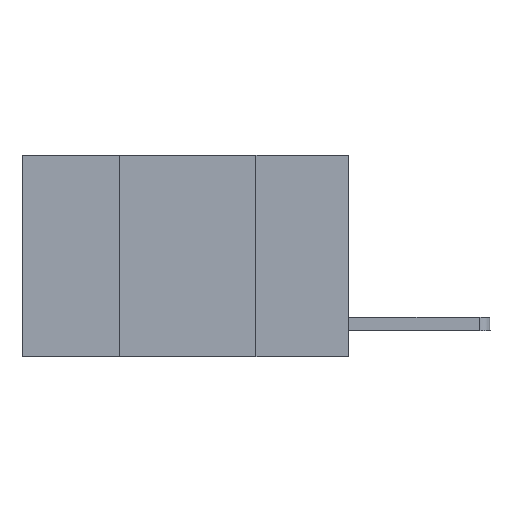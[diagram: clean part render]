
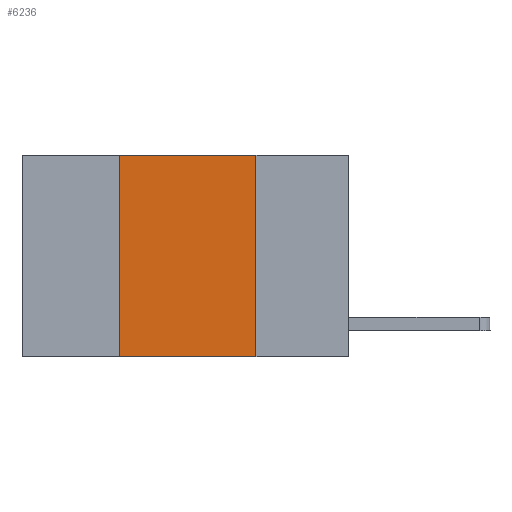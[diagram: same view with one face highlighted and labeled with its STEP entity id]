
A CAD part, left-side view. The second image highlights one B-rep face of the part: STEP entity #6236.
In plain terms, the highlighted planar face has unit normal (-1, 0, 0).
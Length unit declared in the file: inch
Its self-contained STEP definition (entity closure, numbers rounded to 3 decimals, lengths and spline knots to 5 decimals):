
#47 = EDGE_LOOP ( 'NONE', ( #7858, #4166, #7069, #5228 ) ) ;
#303 = VERTEX_POINT ( 'NONE', #2400 ) ;
#845 = DIRECTION ( 'NONE',  ( 1., 0., 0. ) ) ;
#925 = CARTESIAN_POINT ( 'NONE',  ( 0., 0.6, -0.37 ) ) ;
#1009 = CARTESIAN_POINT ( 'NONE',  ( 0., 0.42, 0. ) ) ;
#1465 = LINE ( 'NONE', #1009, #1883 ) ;
#1651 = CARTESIAN_POINT ( 'NONE',  ( 0., 0.6, 0. ) ) ;
#1883 = VECTOR ( 'NONE', #2258, 39.37008 ) ;
#2028 = CARTESIAN_POINT ( 'NONE',  ( 0., 0.17, -0.37 ) ) ;
#2089 = CARTESIAN_POINT ( 'NONE',  ( 0., 0.6, 0. ) ) ;
#2258 = DIRECTION ( 'NONE',  ( 0., 0., 1. ) ) ;
#2332 = DIRECTION ( 'NONE',  ( 0., -1., 0. ) ) ;
#2400 = CARTESIAN_POINT ( 'NONE',  ( 0., 0.42, 0. ) ) ;
#2790 = AXIS2_PLACEMENT_3D ( 'NONE', #2089, #845, #4653 ) ;
#2887 = LINE ( 'NONE', #925, #5223 ) ;
#3063 = CARTESIAN_POINT ( 'NONE',  ( 0., 0.17, 0. ) ) ;
#3121 = VECTOR ( 'NONE', #2332, 39.37008 ) ;
#3943 = VERTEX_POINT ( 'NONE', #6285 ) ;
#4124 = VECTOR ( 'NONE', #5665, 39.37008 ) ;
#4166 = ORIENTED_EDGE ( 'NONE', *, *, #5594, .F. ) ;
#4643 = EDGE_CURVE ( 'NONE', #5069, #7092, #4863, .T. ) ;
#4653 = DIRECTION ( 'NONE',  ( 0., 0., -1. ) ) ;
#4863 = LINE ( 'NONE', #3063, #4124 ) ;
#4965 = EDGE_CURVE ( 'NONE', #3943, #7092, #2887, .T. ) ;
#4993 = EDGE_CURVE ( 'NONE', #3943, #303, #1465, .T. ) ;
#5069 = VERTEX_POINT ( 'NONE', #5512 ) ;
#5223 = VECTOR ( 'NONE', #7253, 39.37008 ) ;
#5228 = ORIENTED_EDGE ( 'NONE', *, *, #4965, .T. ) ;
#5268 = FACE_OUTER_BOUND ( 'NONE', #47, .T. ) ;
#5512 = CARTESIAN_POINT ( 'NONE',  ( 0., 0.17, 0. ) ) ;
#5594 = EDGE_CURVE ( 'NONE', #303, #5069, #7983, .T. ) ;
#5665 = DIRECTION ( 'NONE',  ( 0., 0., -1. ) ) ;
#6236 = ADVANCED_FACE ( 'NONE', ( #5268 ), #7748, .F. ) ;
#6285 = CARTESIAN_POINT ( 'NONE',  ( 0., 0.42, -0.37 ) ) ;
#7069 = ORIENTED_EDGE ( 'NONE', *, *, #4993, .F. ) ;
#7092 = VERTEX_POINT ( 'NONE', #2028 ) ;
#7253 = DIRECTION ( 'NONE',  ( 0., -1., 0. ) ) ;
#7748 = PLANE ( 'NONE',  #2790 ) ;
#7858 = ORIENTED_EDGE ( 'NONE', *, *, #4643, .F. ) ;
#7983 = LINE ( 'NONE', #1651, #3121 ) ;
